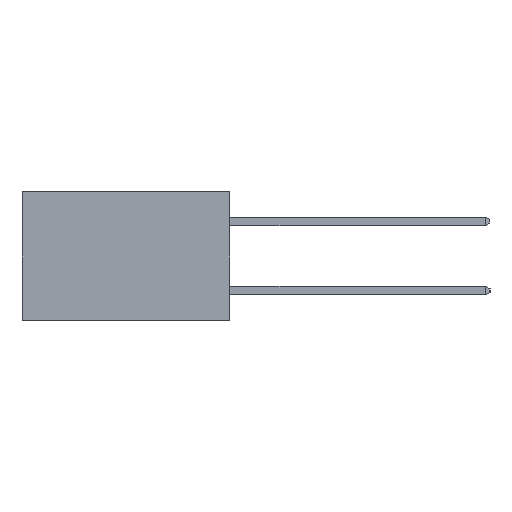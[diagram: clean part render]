
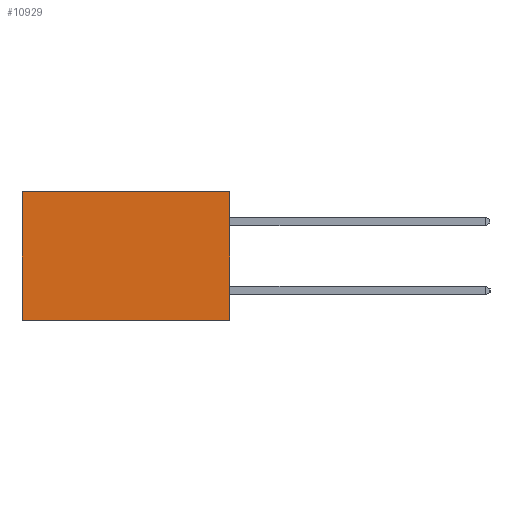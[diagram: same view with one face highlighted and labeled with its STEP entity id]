
A CAD part, left-side view. The second image highlights one B-rep face of the part: STEP entity #10929.
In plain terms, the highlighted planar face has unit normal (-1, 0, 0).
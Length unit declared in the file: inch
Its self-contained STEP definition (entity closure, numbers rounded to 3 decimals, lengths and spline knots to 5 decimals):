
#518 = ORIENTED_EDGE ( 'NONE', *, *, #21210, .T. ) ;
#1264 = EDGE_LOOP ( 'NONE', ( #21968, #21375, #14587, #518 ) ) ;
#1504 = DIRECTION ( 'NONE',  ( 0., 1., 0. ) ) ;
#2379 = DIRECTION ( 'NONE',  ( 0., 0., -1. ) ) ;
#2887 = VECTOR ( 'NONE', #24384, 39.37008 ) ;
#3785 = VERTEX_POINT ( 'NONE', #24246 ) ;
#5162 = VECTOR ( 'NONE', #2379, 39.37008 ) ;
#5867 = CARTESIAN_POINT ( 'NONE',  ( 0.2615, 0.6, -0.37 ) ) ;
#5957 = VERTEX_POINT ( 'NONE', #5867 ) ;
#5972 = DIRECTION ( 'NONE',  ( 0., 0., -1. ) ) ;
#7105 = VECTOR ( 'NONE', #10148, 39.37008 ) ;
#7711 = LINE ( 'NONE', #23161, #7105 ) ;
#8040 = LINE ( 'NONE', #13340, #2887 ) ;
#9261 = VECTOR ( 'NONE', #1504, 39.37008 ) ;
#10148 = DIRECTION ( 'NONE',  ( 0., 1., 0. ) ) ;
#10196 = EDGE_CURVE ( 'NONE', #3785, #22843, #8040, .T. ) ;
#10929 = ADVANCED_FACE ( 'NONE', ( #17241 ), #13650, .F. ) ;
#10961 = LINE ( 'NONE', #21303, #5162 ) ;
#12176 = VERTEX_POINT ( 'NONE', #16964 ) ;
#13340 = CARTESIAN_POINT ( 'NONE',  ( 0.2615, 0., -0.37 ) ) ;
#13650 = PLANE ( 'NONE',  #20363 ) ;
#14345 = LINE ( 'NONE', #16876, #9261 ) ;
#14587 = ORIENTED_EDGE ( 'NONE', *, *, #10196, .F. ) ;
#15560 = CARTESIAN_POINT ( 'NONE',  ( 0.2615, 0., -0.37 ) ) ;
#15801 = CARTESIAN_POINT ( 'NONE',  ( 0.2615, 0., -0.37 ) ) ;
#16876 = CARTESIAN_POINT ( 'NONE',  ( 0.2615, 0., -0.37 ) ) ;
#16964 = CARTESIAN_POINT ( 'NONE',  ( 0.2615, 0.6, 0. ) ) ;
#17241 = FACE_OUTER_BOUND ( 'NONE', #1264, .T. ) ;
#17414 = DIRECTION ( 'NONE',  ( 1., 0., 0. ) ) ;
#17616 = EDGE_CURVE ( 'NONE', #12176, #5957, #10961, .T. ) ;
#20363 = AXIS2_PLACEMENT_3D ( 'NONE', #15560, #17414, #5972 ) ;
#20926 = EDGE_CURVE ( 'NONE', #22843, #5957, #14345, .T. ) ;
#21210 = EDGE_CURVE ( 'NONE', #3785, #12176, #7711, .T. ) ;
#21303 = CARTESIAN_POINT ( 'NONE',  ( 0.2615, 0.6, -0.37 ) ) ;
#21375 = ORIENTED_EDGE ( 'NONE', *, *, #20926, .F. ) ;
#21968 = ORIENTED_EDGE ( 'NONE', *, *, #17616, .T. ) ;
#22843 = VERTEX_POINT ( 'NONE', #15801 ) ;
#23161 = CARTESIAN_POINT ( 'NONE',  ( 0.2615, 0., 0. ) ) ;
#24246 = CARTESIAN_POINT ( 'NONE',  ( 0.2615, 0., 0. ) ) ;
#24384 = DIRECTION ( 'NONE',  ( 0., 0., -1. ) ) ;
